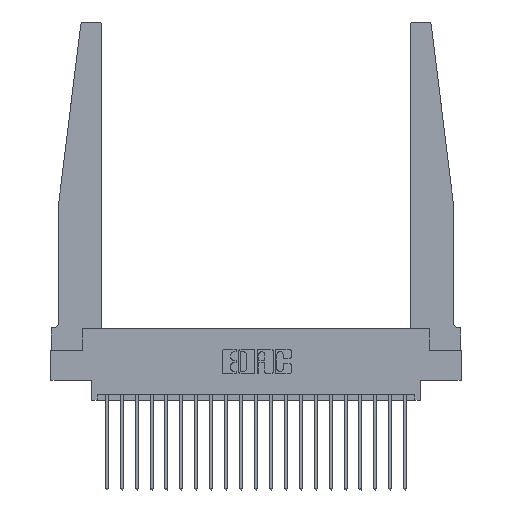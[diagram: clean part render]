
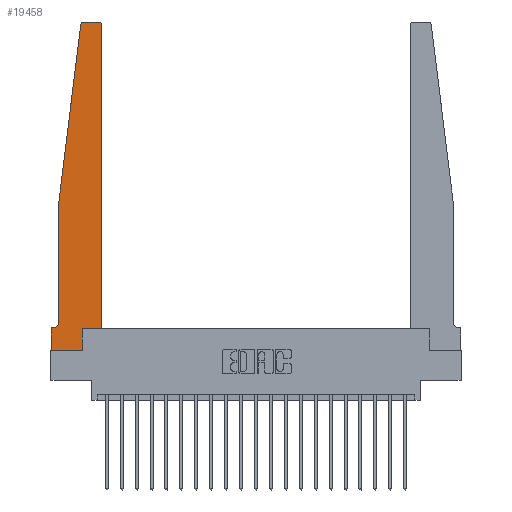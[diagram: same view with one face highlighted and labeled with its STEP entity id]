
A CAD part, top view. The second image highlights one B-rep face of the part: STEP entity #19458.
In plain terms, the highlighted planar face has unit normal (0, 0, 1).
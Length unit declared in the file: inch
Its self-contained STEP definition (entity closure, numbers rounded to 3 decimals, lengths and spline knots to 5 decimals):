
#41 = DIRECTION ( 'NONE',  ( 1., 0., 0. ) ) ;
#56 = DIRECTION ( 'NONE',  ( 0., 1., 0. ) ) ;
#286 = ORIENTED_EDGE ( 'NONE', *, *, #11685, .T. ) ;
#895 = VECTOR ( 'NONE', #7010, 39.37008 ) ;
#1031 = ORIENTED_EDGE ( 'NONE', *, *, #10510, .T. ) ;
#1218 = DIRECTION ( 'NONE',  ( 1., 0., 0. ) ) ;
#1439 = DIRECTION ( 'NONE',  ( 0., 1., 0. ) ) ;
#1645 = ORIENTED_EDGE ( 'NONE', *, *, #14332, .T. ) ;
#1662 = CARTESIAN_POINT ( 'NONE',  ( 0.425, 0.18, 0.37 ) ) ;
#1689 = VERTEX_POINT ( 'NONE', #12817 ) ;
#1900 = VERTEX_POINT ( 'NONE', #3634 ) ;
#2317 = DIRECTION ( 'NONE',  ( 0., 0., 1. ) ) ;
#2334 = EDGE_LOOP ( 'NONE', ( #10956, #15749, #21234, #4078, #11638, #286, #1031, #1645, #17329, #4496, #17446, #12722 ) ) ;
#2365 = CARTESIAN_POINT ( 'NONE',  ( 0., 0.1875, 0.37 ) ) ;
#3134 = AXIS2_PLACEMENT_3D ( 'NONE', #12213, #2317, #13914 ) ;
#3297 = VERTEX_POINT ( 'NONE', #3798 ) ;
#3324 = EDGE_CURVE ( 'NONE', #11637, #3297, #9706, .T. ) ;
#3416 = DIRECTION ( 'NONE',  ( 0., -1., 0. ) ) ;
#3572 = LINE ( 'NONE', #14073, #6898 ) ;
#3634 = CARTESIAN_POINT ( 'NONE',  ( 0.425, 2.72, 0.37 ) ) ;
#3655 = EDGE_CURVE ( 'NONE', #16204, #4904, #12793, .T. ) ;
#3798 = CARTESIAN_POINT ( 'NONE',  ( 0.065, 1.25, 0.37 ) ) ;
#3886 = DIRECTION ( 'NONE',  ( 0., -1., 0. ) ) ;
#4023 = DIRECTION ( 'NONE',  ( 0., 0., 1. ) ) ;
#4078 = ORIENTED_EDGE ( 'NONE', *, *, #11385, .T. ) ;
#4136 = DIRECTION ( 'NONE',  ( -1., 0., 0. ) ) ;
#4476 = LINE ( 'NONE', #8281, #21075 ) ;
#4496 = ORIENTED_EDGE ( 'NONE', *, *, #19156, .T. ) ;
#4534 = CIRCLE ( 'NONE', #3134, 0.03 ) ;
#4551 = CARTESIAN_POINT ( 'NONE',  ( 0.015, 0.2375, 0.37 ) ) ;
#4638 = VECTOR ( 'NONE', #3416, 39.37008 ) ;
#4904 = VERTEX_POINT ( 'NONE', #16331 ) ;
#5843 = EDGE_CURVE ( 'NONE', #17963, #11637, #4534, .T. ) ;
#6191 = VERTEX_POINT ( 'NONE', #6400 ) ;
#6205 = DIRECTION ( 'NONE',  ( -1., 0., 0. ) ) ;
#6400 = CARTESIAN_POINT ( 'NONE',  ( 0.2605, 0., 0.37 ) ) ;
#6511 = CARTESIAN_POINT ( 'NONE',  ( 0.065, 0.2375, 0.37 ) ) ;
#6898 = VECTOR ( 'NONE', #4136, 39.37008 ) ;
#7010 = DIRECTION ( 'NONE',  ( -0.122, -0.992, 0. ) ) ;
#8281 = CARTESIAN_POINT ( 'NONE',  ( 0.425, 0.18, 0.37 ) ) ;
#8967 = VECTOR ( 'NONE', #56, 39.37008 ) ;
#9034 = VECTOR ( 'NONE', #19842, 39.37008 ) ;
#9233 = CARTESIAN_POINT ( 'NONE',  ( 0., 0., 0.37 ) ) ;
#9706 = LINE ( 'NONE', #10451, #895 ) ;
#9737 = CARTESIAN_POINT ( 'NONE',  ( 0.24675, 2.72367, 0.37 ) ) ;
#9886 = CARTESIAN_POINT ( 'NONE',  ( 0.065, 0.1875, 0.37 ) ) ;
#9976 = CARTESIAN_POINT ( 'NONE',  ( 0.2605, 0.18, 0.37 ) ) ;
#10348 = VECTOR ( 'NONE', #3886, 39.37008 ) ;
#10451 = CARTESIAN_POINT ( 'NONE',  ( 0.065, 1.25, 0.37 ) ) ;
#10510 = EDGE_CURVE ( 'NONE', #16676, #19569, #12417, .T. ) ;
#10956 = ORIENTED_EDGE ( 'NONE', *, *, #12760, .T. ) ;
#11125 = DIRECTION ( 'NONE',  ( 0., 0., 1. ) ) ;
#11385 = EDGE_CURVE ( 'NONE', #3297, #16204, #18705, .T. ) ;
#11637 = VERTEX_POINT ( 'NONE', #9737 ) ;
#11638 = ORIENTED_EDGE ( 'NONE', *, *, #3655, .T. ) ;
#11685 = EDGE_CURVE ( 'NONE', #4904, #16676, #13986, .T. ) ;
#11718 = CARTESIAN_POINT ( 'NONE',  ( 0., 0., 0.37 ) ) ;
#11742 = CARTESIAN_POINT ( 'NONE',  ( 0.395, 2.75, 0.37 ) ) ;
#11803 = DIRECTION ( 'NONE',  ( 1., 0., 0. ) ) ;
#12213 = CARTESIAN_POINT ( 'NONE',  ( 0.27653, 2.72, 0.37 ) ) ;
#12267 = PLANE ( 'NONE',  #17406 ) ;
#12417 = LINE ( 'NONE', #11718, #4638 ) ;
#12606 = CIRCLE ( 'NONE', #14900, 0.03 ) ;
#12722 = ORIENTED_EDGE ( 'NONE', *, *, #12926, .T. ) ;
#12760 = EDGE_CURVE ( 'NONE', #17566, #17963, #3572, .T. ) ;
#12782 = VECTOR ( 'NONE', #1439, 39.37008 ) ;
#12793 = CIRCLE ( 'NONE', #20206, 0.05 ) ;
#12817 = CARTESIAN_POINT ( 'NONE',  ( 0.2605, 0.18, 0.37 ) ) ;
#12855 = LINE ( 'NONE', #9976, #8967 ) ;
#12926 = EDGE_CURVE ( 'NONE', #1900, #17566, #12606, .T. ) ;
#13140 = EDGE_CURVE ( 'NONE', #6191, #1689, #12855, .T. ) ;
#13502 = CARTESIAN_POINT ( 'NONE',  ( 0., 0., 0.37 ) ) ;
#13914 = DIRECTION ( 'NONE',  ( 1., 0., 0. ) ) ;
#13986 = LINE ( 'NONE', #9886, #9034 ) ;
#14073 = CARTESIAN_POINT ( 'NONE',  ( 0.25, 2.75, 0.37 ) ) ;
#14142 = LINE ( 'NONE', #13502, #18583 ) ;
#14332 = EDGE_CURVE ( 'NONE', #19569, #6191, #14142, .T. ) ;
#14900 = AXIS2_PLACEMENT_3D ( 'NONE', #21086, #11125, #1218 ) ;
#15519 = CARTESIAN_POINT ( 'NONE',  ( 0.065, 1.25, 0.37 ) ) ;
#15593 = CARTESIAN_POINT ( 'NONE',  ( 0.425, 0.18, 0.37 ) ) ;
#15661 = DIRECTION ( 'NONE',  ( 1., 0., 0. ) ) ;
#15749 = ORIENTED_EDGE ( 'NONE', *, *, #5843, .T. ) ;
#15942 = FACE_OUTER_BOUND ( 'NONE', #2334, .T. ) ;
#16204 = VERTEX_POINT ( 'NONE', #6511 ) ;
#16240 = DIRECTION ( 'NONE',  ( 0., 0., -1. ) ) ;
#16331 = CARTESIAN_POINT ( 'NONE',  ( 0.015, 0.1875, 0.37 ) ) ;
#16676 = VERTEX_POINT ( 'NONE', #19375 ) ;
#17115 = VERTEX_POINT ( 'NONE', #15593 ) ;
#17294 = LINE ( 'NONE', #1662, #12782 ) ;
#17329 = ORIENTED_EDGE ( 'NONE', *, *, #13140, .T. ) ;
#17406 = AXIS2_PLACEMENT_3D ( 'NONE', #2365, #4023, #15661 ) ;
#17446 = ORIENTED_EDGE ( 'NONE', *, *, #18711, .T. ) ;
#17566 = VERTEX_POINT ( 'NONE', #11742 ) ;
#17841 = CARTESIAN_POINT ( 'NONE',  ( 0.27653, 2.75, 0.37 ) ) ;
#17963 = VERTEX_POINT ( 'NONE', #17841 ) ;
#18583 = VECTOR ( 'NONE', #11803, 39.37008 ) ;
#18705 = LINE ( 'NONE', #15519, #10348 ) ;
#18711 = EDGE_CURVE ( 'NONE', #17115, #1900, #17294, .T. ) ;
#19156 = EDGE_CURVE ( 'NONE', #1689, #17115, #4476, .T. ) ;
#19375 = CARTESIAN_POINT ( 'NONE',  ( 0., 0.1875, 0.37 ) ) ;
#19458 = ADVANCED_FACE ( 'NONE', ( #15942 ), #12267, .T. ) ;
#19569 = VERTEX_POINT ( 'NONE', #9233 ) ;
#19842 = DIRECTION ( 'NONE',  ( -1., 0., 0. ) ) ;
#20206 = AXIS2_PLACEMENT_3D ( 'NONE', #4551, #16240, #6205 ) ;
#21075 = VECTOR ( 'NONE', #41, 39.37008 ) ;
#21086 = CARTESIAN_POINT ( 'NONE',  ( 0.395, 2.72, 0.37 ) ) ;
#21234 = ORIENTED_EDGE ( 'NONE', *, *, #3324, .T. ) ;
